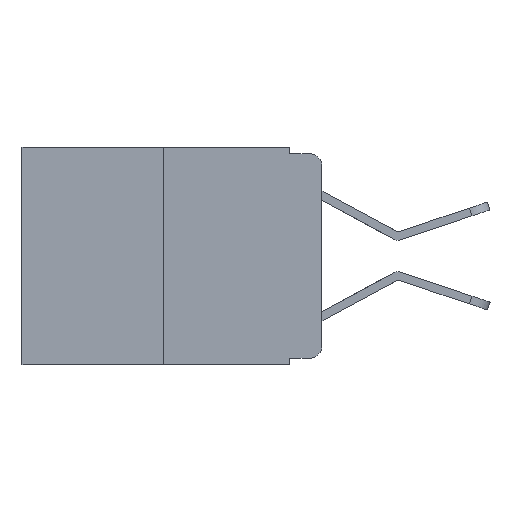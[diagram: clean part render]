
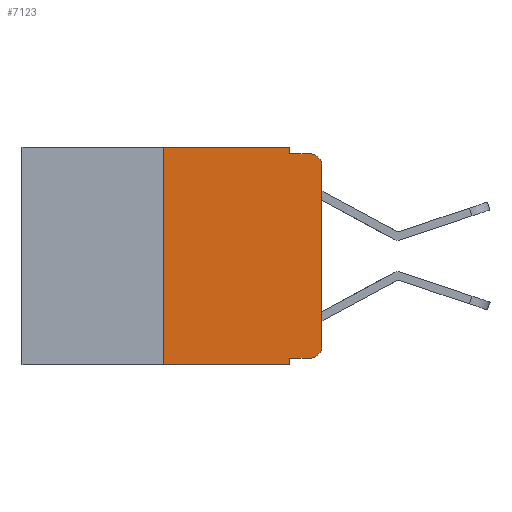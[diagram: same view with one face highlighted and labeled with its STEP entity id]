
A CAD part, left-side view. The second image highlights one B-rep face of the part: STEP entity #7123.
In plain terms, the highlighted planar face has unit normal (-1, 0, 0).
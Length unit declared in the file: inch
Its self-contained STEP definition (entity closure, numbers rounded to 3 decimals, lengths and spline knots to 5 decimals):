
#79 = VERTEX_POINT ( 'NONE', #10159 ) ;
#82 = CARTESIAN_POINT ( 'NONE',  ( 0., 0.473, 0. ) ) ;
#399 = VERTEX_POINT ( 'NONE', #11180 ) ;
#428 = ORIENTED_EDGE ( 'NONE', *, *, #1431, .F. ) ;
#456 = VECTOR ( 'NONE', #11334, 39.37008 ) ;
#491 = VECTOR ( 'NONE', #5893, 39.37008 ) ;
#643 = DIRECTION ( 'NONE',  ( 0., -1., 0. ) ) ;
#684 = ORIENTED_EDGE ( 'NONE', *, *, #9991, .F. ) ;
#710 = ORIENTED_EDGE ( 'NONE', *, *, #10784, .T. ) ;
#805 = EDGE_CURVE ( 'NONE', #6902, #4150, #11710, .T. ) ;
#838 = VERTEX_POINT ( 'NONE', #1514 ) ;
#976 = CARTESIAN_POINT ( 'NONE',  ( 0., 0.051, 0. ) ) ;
#983 = VECTOR ( 'NONE', #3734, 39.37008 ) ;
#1014 = CARTESIAN_POINT ( 'NONE',  ( 0., 0.051, -0.343 ) ) ;
#1180 = VERTEX_POINT ( 'NONE', #2090 ) ;
#1431 = EDGE_CURVE ( 'NONE', #79, #11979, #7373, .T. ) ;
#1514 = CARTESIAN_POINT ( 'NONE',  ( 0., 0.02, -0.333 ) ) ;
#1730 = DIRECTION ( 'NONE',  ( 0., 0., 1. ) ) ;
#1757 = ORIENTED_EDGE ( 'NONE', *, *, #4123, .F. ) ;
#1891 = CARTESIAN_POINT ( 'NONE',  ( 0., 0.473, 0. ) ) ;
#2090 = CARTESIAN_POINT ( 'NONE',  ( 0., 0.02, -0.01 ) ) ;
#2557 = EDGE_CURVE ( 'NONE', #4735, #399, #4271, .T. ) ;
#2711 = VECTOR ( 'NONE', #4888, 39.37008 ) ;
#3141 = EDGE_CURVE ( 'NONE', #838, #4735, #9705, .T. ) ;
#3299 = ORIENTED_EDGE ( 'NONE', *, *, #9452, .F. ) ;
#3492 = CARTESIAN_POINT ( 'NONE',  ( 0., 0., 0. ) ) ;
#3734 = DIRECTION ( 'NONE',  ( 0., 0., -1. ) ) ;
#3857 = CARTESIAN_POINT ( 'NONE',  ( 0., 0.051, -0.333 ) ) ;
#3893 = LINE ( 'NONE', #6698, #491 ) ;
#3966 = DIRECTION ( 'NONE',  ( 0., 0., -1. ) ) ;
#4012 = LINE ( 'NONE', #3857, #456 ) ;
#4102 = ORIENTED_EDGE ( 'NONE', *, *, #7048, .T. ) ;
#4123 = EDGE_CURVE ( 'NONE', #9173, #4150, #5995, .T. ) ;
#4150 = VERTEX_POINT ( 'NONE', #1014 ) ;
#4192 = ORIENTED_EDGE ( 'NONE', *, *, #3141, .T. ) ;
#4271 = LINE ( 'NONE', #3492, #8677 ) ;
#4735 = VERTEX_POINT ( 'NONE', #7651 ) ;
#4758 = CARTESIAN_POINT ( 'NONE',  ( 0., 0.25, 0. ) ) ;
#4888 = DIRECTION ( 'NONE',  ( 0., -1., 0. ) ) ;
#4899 = VECTOR ( 'NONE', #5698, 39.37008 ) ;
#4986 = VERTEX_POINT ( 'NONE', #6315 ) ;
#5194 = LINE ( 'NONE', #6750, #2711 ) ;
#5659 = DIRECTION ( 'NONE',  ( 0., 0., -1. ) ) ;
#5698 = DIRECTION ( 'NONE',  ( 0., 0., 1. ) ) ;
#5806 = ORIENTED_EDGE ( 'NONE', *, *, #9401, .F. ) ;
#5893 = DIRECTION ( 'NONE',  ( 0., 0., -1. ) ) ;
#5995 = LINE ( 'NONE', #976, #983 ) ;
#6315 = CARTESIAN_POINT ( 'NONE',  ( 0., 0.051, -0.01 ) ) ;
#6554 = PLANE ( 'NONE',  #11789 ) ;
#6698 = CARTESIAN_POINT ( 'NONE',  ( 0., 0.051, 0. ) ) ;
#6750 = CARTESIAN_POINT ( 'NONE',  ( 0., 0.051, -0.01 ) ) ;
#6810 = VECTOR ( 'NONE', #643, 39.37008 ) ;
#6902 = VERTEX_POINT ( 'NONE', #9039 ) ;
#7048 = EDGE_CURVE ( 'NONE', #399, #1180, #12090, .T. ) ;
#7105 = CARTESIAN_POINT ( 'NONE',  ( 0., 0.473, -0.343 ) ) ;
#7123 = ADVANCED_FACE ( 'NONE', ( #8797 ), #6554, .F. ) ;
#7373 = LINE ( 'NONE', #82, #10195 ) ;
#7478 = DIRECTION ( 'NONE',  ( 0., 0., -1. ) ) ;
#7544 = LINE ( 'NONE', #4758, #4899 ) ;
#7651 = CARTESIAN_POINT ( 'NONE',  ( 0., 0., -0.313 ) ) ;
#8462 = DIRECTION ( 'NONE',  ( 1., 0., 0. ) ) ;
#8515 = EDGE_LOOP ( 'NONE', ( #10025, #4102, #3299, #5806, #428, #684, #8789, #1757, #710, #4192 ) ) ;
#8677 = VECTOR ( 'NONE', #1730, 39.37008 ) ;
#8789 = ORIENTED_EDGE ( 'NONE', *, *, #805, .T. ) ;
#8797 = FACE_OUTER_BOUND ( 'NONE', #8515, .T. ) ;
#9039 = CARTESIAN_POINT ( 'NONE',  ( 0., 0.25, -0.343 ) ) ;
#9173 = VERTEX_POINT ( 'NONE', #10222 ) ;
#9401 = EDGE_CURVE ( 'NONE', #11979, #4986, #3893, .T. ) ;
#9452 = EDGE_CURVE ( 'NONE', #4986, #1180, #5194, .T. ) ;
#9705 = CIRCLE ( 'NONE', #10875, 0.02 ) ;
#9991 = EDGE_CURVE ( 'NONE', #6902, #79, #7544, .T. ) ;
#10025 = ORIENTED_EDGE ( 'NONE', *, *, #2557, .T. ) ;
#10148 = CARTESIAN_POINT ( 'NONE',  ( 0., 0.051, 0. ) ) ;
#10159 = CARTESIAN_POINT ( 'NONE',  ( 0., 0.25, 0. ) ) ;
#10195 = VECTOR ( 'NONE', #11526, 39.37008 ) ;
#10197 = CARTESIAN_POINT ( 'NONE',  ( 0., 0.02, -0.313 ) ) ;
#10222 = CARTESIAN_POINT ( 'NONE',  ( 0., 0.051, -0.333 ) ) ;
#10331 = CARTESIAN_POINT ( 'NONE',  ( 0., 0.02, -0.03 ) ) ;
#10784 = EDGE_CURVE ( 'NONE', #9173, #838, #4012, .T. ) ;
#10875 = AXIS2_PLACEMENT_3D ( 'NONE', #10197, #11743, #3966 ) ;
#11180 = CARTESIAN_POINT ( 'NONE',  ( 0., 0., -0.03 ) ) ;
#11212 = DIRECTION ( 'NONE',  ( -1., 0., 0. ) ) ;
#11334 = DIRECTION ( 'NONE',  ( 0., -1., 0. ) ) ;
#11367 = AXIS2_PLACEMENT_3D ( 'NONE', #10331, #11212, #7478 ) ;
#11526 = DIRECTION ( 'NONE',  ( 0., -1., 0. ) ) ;
#11710 = LINE ( 'NONE', #7105, #6810 ) ;
#11743 = DIRECTION ( 'NONE',  ( -1., 0., 0. ) ) ;
#11789 = AXIS2_PLACEMENT_3D ( 'NONE', #1891, #8462, #5659 ) ;
#11979 = VERTEX_POINT ( 'NONE', #10148 ) ;
#12090 = CIRCLE ( 'NONE', #11367, 0.02 ) ;
